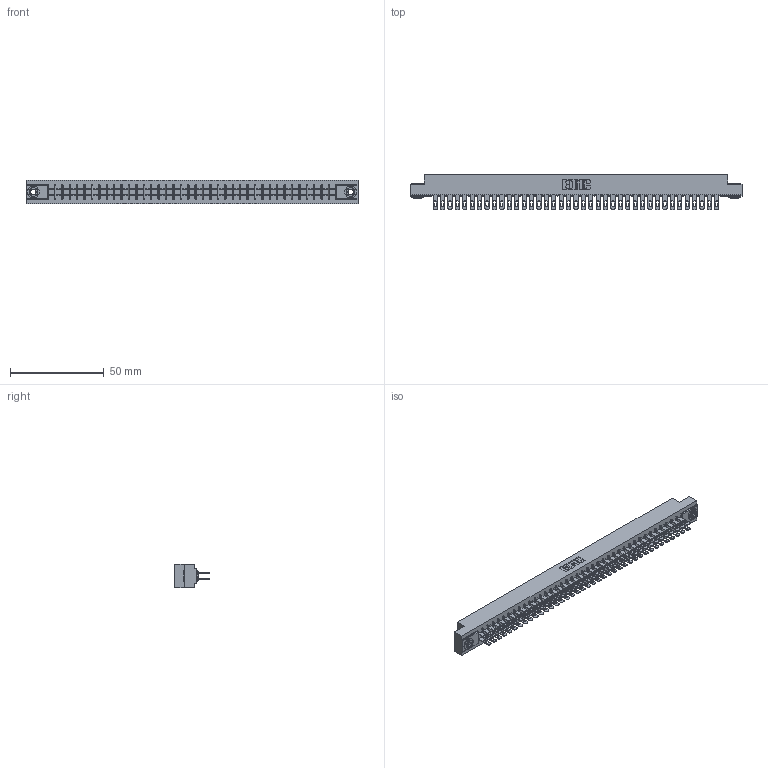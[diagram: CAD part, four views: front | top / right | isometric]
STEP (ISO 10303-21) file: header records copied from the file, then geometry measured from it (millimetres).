
FILE_DESCRIPTION (( 'STEP AP203' ), '1' );
FILE_NAME ('305-078-500-503.STEP', '2019-09-10T08:39:34', ( '' ), ( '' ), 'SwSTEP 2.0', 'SolidWorks 2016', '' );
FILE_SCHEMA (( 'CONFIG_CONTROL_DESIGN' ));
Length unit declared in the file: inch
Products named in the file (4): 305-078-500-503; 305 Part_.156 Dia; 345-250-002_345-250-002-102; 305-290-001_500
Assembly tree (81 placements, depth 2):
  305-078-500-503
    305 Part_.156 Dia
    305-290-001_500  x78
    345-250-002_345-250-002-102  x2
Bounding box: 177.55 x 18.85 x 12.7 mm (x, y, z)
Volume: 18207.4 mm3; surface area: 25736.4 mm2
Topology: 81 solids, 81 shells, 4068 faces, 11621 edges, 7534 vertices
Faces by surface type: plane 2276, cylinder 1628, sphere 156, cone 8
Entity records: 43679 total; most frequent: CARTESIAN_POINT 7208, ORIENTED_EDGE 7146, DIRECTION 6993, EDGE_CURVE 3573, LINE 2875, VECTOR 2875, VERTEX_POINT 2274, AXIS2_PLACEMENT_3D 2059
